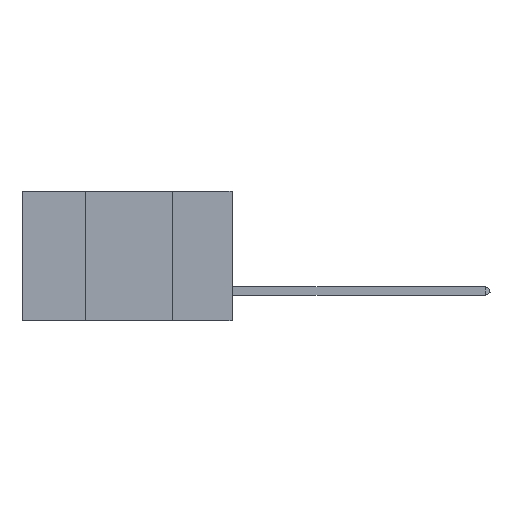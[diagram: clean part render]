
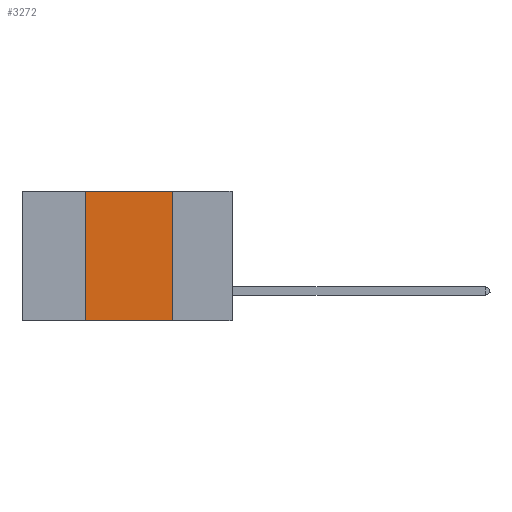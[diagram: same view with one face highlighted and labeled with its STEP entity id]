
A CAD part, left-side view. The second image highlights one B-rep face of the part: STEP entity #3272.
In plain terms, the highlighted planar face has unit normal (-1, 0, 0).
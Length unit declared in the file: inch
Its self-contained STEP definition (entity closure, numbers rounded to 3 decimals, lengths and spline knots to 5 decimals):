
#69 = ORIENTED_EDGE ( 'NONE', *, *, #18779, .F. ) ;
#235 = LINE ( 'NONE', #10903, #11969 ) ;
#385 = EDGE_CURVE ( 'NONE', #8766, #16314, #1831, .T. ) ;
#718 = VERTEX_POINT ( 'NONE', #2440 ) ;
#1175 = EDGE_CURVE ( 'NONE', #8766, #718, #10888, .T. ) ;
#1392 = FACE_OUTER_BOUND ( 'NONE', #15738, .T. ) ;
#1831 = LINE ( 'NONE', #21553, #21702 ) ;
#2440 = CARTESIAN_POINT ( 'NONE',  ( 0., 0.17, -0.37 ) ) ;
#3049 = VECTOR ( 'NONE', #24067, 39.37008 ) ;
#3272 = ADVANCED_FACE ( 'NONE', ( #1392 ), #11983, .F. ) ;
#4543 = CARTESIAN_POINT ( 'NONE',  ( 0., 0.17, 0. ) ) ;
#5805 = CARTESIAN_POINT ( 'NONE',  ( 0., 0.17, 0. ) ) ;
#6356 = CARTESIAN_POINT ( 'NONE',  ( 0., 0.6, 0. ) ) ;
#6496 = DIRECTION ( 'NONE',  ( 0., 0., -1. ) ) ;
#7907 = DIRECTION ( 'NONE',  ( 0., 0., 1. ) ) ;
#8578 = CARTESIAN_POINT ( 'NONE',  ( 0., 0.42, 0. ) ) ;
#8766 = VERTEX_POINT ( 'NONE', #14689 ) ;
#8971 = ORIENTED_EDGE ( 'NONE', *, *, #11948, .F. ) ;
#10574 = VECTOR ( 'NONE', #6496, 39.37008 ) ;
#10888 = LINE ( 'NONE', #12961, #3049 ) ;
#10903 = CARTESIAN_POINT ( 'NONE',  ( 0., 0.6, 0. ) ) ;
#11373 = AXIS2_PLACEMENT_3D ( 'NONE', #6356, #23730, #21081 ) ;
#11948 = EDGE_CURVE ( 'NONE', #13149, #718, #14432, .T. ) ;
#11969 = VECTOR ( 'NONE', #22238, 39.37008 ) ;
#11983 = PLANE ( 'NONE',  #11373 ) ;
#12961 = CARTESIAN_POINT ( 'NONE',  ( 0., 0.6, -0.37 ) ) ;
#13149 = VERTEX_POINT ( 'NONE', #5805 ) ;
#14351 = ORIENTED_EDGE ( 'NONE', *, *, #1175, .T. ) ;
#14432 = LINE ( 'NONE', #4543, #10574 ) ;
#14689 = CARTESIAN_POINT ( 'NONE',  ( 0., 0.42, -0.37 ) ) ;
#15738 = EDGE_LOOP ( 'NONE', ( #8971, #69, #24097, #14351 ) ) ;
#16314 = VERTEX_POINT ( 'NONE', #8578 ) ;
#18779 = EDGE_CURVE ( 'NONE', #16314, #13149, #235, .T. ) ;
#21081 = DIRECTION ( 'NONE',  ( 0., 0., -1. ) ) ;
#21553 = CARTESIAN_POINT ( 'NONE',  ( 0., 0.42, 0. ) ) ;
#21702 = VECTOR ( 'NONE', #7907, 39.37008 ) ;
#22238 = DIRECTION ( 'NONE',  ( 0., -1., 0. ) ) ;
#23730 = DIRECTION ( 'NONE',  ( 1., 0., 0. ) ) ;
#24067 = DIRECTION ( 'NONE',  ( 0., -1., 0. ) ) ;
#24097 = ORIENTED_EDGE ( 'NONE', *, *, #385, .F. ) ;
